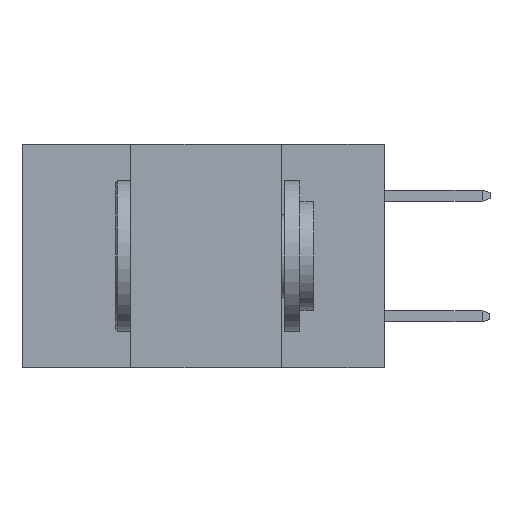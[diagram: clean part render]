
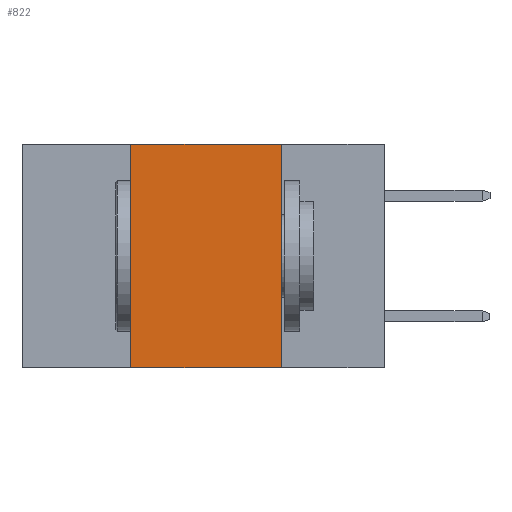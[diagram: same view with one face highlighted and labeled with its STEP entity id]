
A CAD part, left-side view. The second image highlights one B-rep face of the part: STEP entity #822.
In plain terms, the highlighted planar face has unit normal (-1, 0, 0).
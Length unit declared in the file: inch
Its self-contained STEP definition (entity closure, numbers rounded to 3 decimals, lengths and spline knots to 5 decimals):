
#38 = EDGE_CURVE ( 'NONE', #12030, #286, #11046, .T. ) ;
#286 = VERTEX_POINT ( 'NONE', #4587 ) ;
#404 = CARTESIAN_POINT ( 'NONE',  ( 0., 0.17, 0. ) ) ;
#822 = ADVANCED_FACE ( 'NONE', ( #11372 ), #5679, .F. ) ;
#1641 = CARTESIAN_POINT ( 'NONE',  ( 0., 0.6, -0.37 ) ) ;
#1817 = ORIENTED_EDGE ( 'NONE', *, *, #8199, .F. ) ;
#2641 = ORIENTED_EDGE ( 'NONE', *, *, #4445, .F. ) ;
#2862 = ORIENTED_EDGE ( 'NONE', *, *, #10016, .F. ) ;
#3057 = VECTOR ( 'NONE', #6705, 39.37008 ) ;
#3175 = ORIENTED_EDGE ( 'NONE', *, *, #38, .T. ) ;
#3326 = DIRECTION ( 'NONE',  ( 0., -1., 0. ) ) ;
#3920 = CARTESIAN_POINT ( 'NONE',  ( 0., 0.6, 0. ) ) ;
#4331 = DIRECTION ( 'NONE',  ( 0., 0., -1. ) ) ;
#4445 = EDGE_CURVE ( 'NONE', #10279, #10461, #4516, .T. ) ;
#4516 = LINE ( 'NONE', #3920, #7251 ) ;
#4587 = CARTESIAN_POINT ( 'NONE',  ( 0., 0.17, -0.37 ) ) ;
#5062 = CARTESIAN_POINT ( 'NONE',  ( 0., 0.6, 0. ) ) ;
#5210 = CARTESIAN_POINT ( 'NONE',  ( 0., 0.17, 0. ) ) ;
#5679 = PLANE ( 'NONE',  #7698 ) ;
#5818 = DIRECTION ( 'NONE',  ( 0., 0., -1. ) ) ;
#5891 = DIRECTION ( 'NONE',  ( 1., 0., 0. ) ) ;
#5898 = VECTOR ( 'NONE', #4331, 39.37008 ) ;
#6143 = LINE ( 'NONE', #6453, #3057 ) ;
#6453 = CARTESIAN_POINT ( 'NONE',  ( 0., 0.42, 0. ) ) ;
#6705 = DIRECTION ( 'NONE',  ( 0., 0., 1. ) ) ;
#7251 = VECTOR ( 'NONE', #3326, 39.37008 ) ;
#7457 = DIRECTION ( 'NONE',  ( 0., -1., 0. ) ) ;
#7698 = AXIS2_PLACEMENT_3D ( 'NONE', #5062, #5891, #5818 ) ;
#8199 = EDGE_CURVE ( 'NONE', #10461, #286, #8784, .T. ) ;
#8528 = CARTESIAN_POINT ( 'NONE',  ( 0., 0.42, 0. ) ) ;
#8784 = LINE ( 'NONE', #404, #5898 ) ;
#9501 = CARTESIAN_POINT ( 'NONE',  ( 0., 0.42, -0.37 ) ) ;
#10016 = EDGE_CURVE ( 'NONE', #12030, #10279, #6143, .T. ) ;
#10279 = VERTEX_POINT ( 'NONE', #8528 ) ;
#10461 = VERTEX_POINT ( 'NONE', #5210 ) ;
#11046 = LINE ( 'NONE', #1641, #11383 ) ;
#11372 = FACE_OUTER_BOUND ( 'NONE', #12230, .T. ) ;
#11383 = VECTOR ( 'NONE', #7457, 39.37008 ) ;
#12030 = VERTEX_POINT ( 'NONE', #9501 ) ;
#12230 = EDGE_LOOP ( 'NONE', ( #1817, #2641, #2862, #3175 ) ) ;
